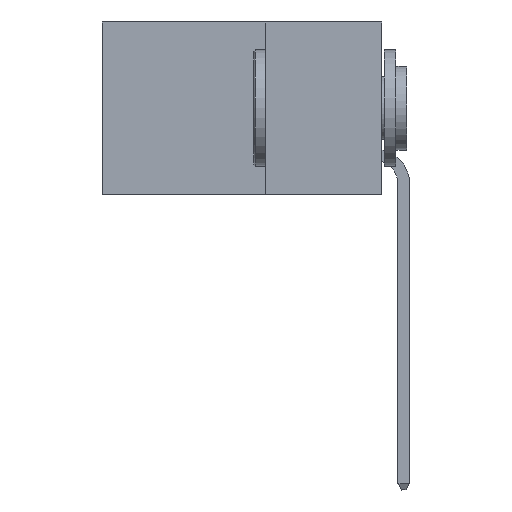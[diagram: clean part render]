
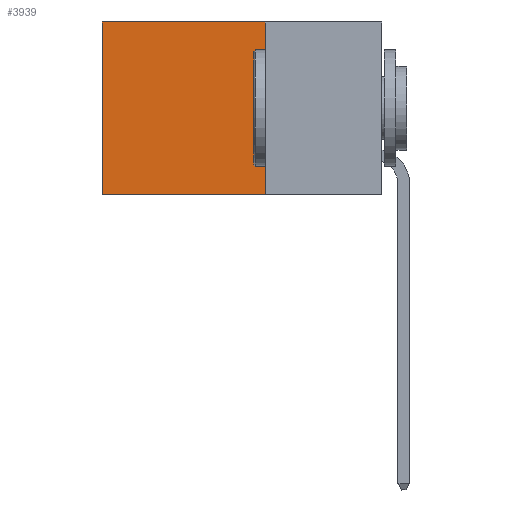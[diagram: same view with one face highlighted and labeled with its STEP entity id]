
A CAD part, left-side view. The second image highlights one B-rep face of the part: STEP entity #3939.
In plain terms, the highlighted planar face has unit normal (-1, 0, 0).
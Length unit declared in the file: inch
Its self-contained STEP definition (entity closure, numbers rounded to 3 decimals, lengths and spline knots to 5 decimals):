
#18 = CARTESIAN_POINT ( 'NONE',  ( 0.2875, 0.25, 0. ) ) ;
#191 = DIRECTION ( 'NONE',  ( 0., 0., -1. ) ) ;
#326 = DIRECTION ( 'NONE',  ( 0., 1., 0. ) ) ;
#1387 = CARTESIAN_POINT ( 'NONE',  ( 0.2875, 0.6, 0. ) ) ;
#1940 = ORIENTED_EDGE ( 'NONE', *, *, #3908, .F. ) ;
#2828 = EDGE_CURVE ( 'NONE', #11890, #6327, #3169, .T. ) ;
#2958 = EDGE_CURVE ( 'NONE', #12188, #11890, #14932, .T. ) ;
#3169 = LINE ( 'NONE', #1387, #8463 ) ;
#3596 = ORIENTED_EDGE ( 'NONE', *, *, #2958, .T. ) ;
#3908 = EDGE_CURVE ( 'NONE', #12188, #13177, #7261, .T. ) ;
#3912 = CARTESIAN_POINT ( 'NONE',  ( 0.2875, 0.6, 0. ) ) ;
#3939 = ADVANCED_FACE ( 'NONE', ( #4134 ), #12779, .F. ) ;
#4134 = FACE_OUTER_BOUND ( 'NONE', #4373, .T. ) ;
#4373 = EDGE_LOOP ( 'NONE', ( #7343, #8391, #1940, #3596 ) ) ;
#4452 = EDGE_CURVE ( 'NONE', #13177, #6327, #12382, .T. ) ;
#5087 = DIRECTION ( 'NONE',  ( 0., 0., -1. ) ) ;
#6280 = VECTOR ( 'NONE', #191, 39.37008 ) ;
#6327 = VERTEX_POINT ( 'NONE', #12019 ) ;
#6412 = CARTESIAN_POINT ( 'NONE',  ( 0.2875, 0.25, 0. ) ) ;
#6485 = VECTOR ( 'NONE', #326, 39.37008 ) ;
#7078 = CARTESIAN_POINT ( 'NONE',  ( 0.2875, 0.25, 0. ) ) ;
#7261 = LINE ( 'NONE', #6412, #6280 ) ;
#7343 = ORIENTED_EDGE ( 'NONE', *, *, #2828, .T. ) ;
#8306 = DIRECTION ( 'NONE',  ( 0., 1., 0. ) ) ;
#8391 = ORIENTED_EDGE ( 'NONE', *, *, #4452, .F. ) ;
#8463 = VECTOR ( 'NONE', #5087, 39.37008 ) ;
#9861 = CARTESIAN_POINT ( 'NONE',  ( 0.2875, 0.25, -0.37 ) ) ;
#10328 = CARTESIAN_POINT ( 'NONE',  ( 0.2875, 0.25, -0.37 ) ) ;
#11086 = AXIS2_PLACEMENT_3D ( 'NONE', #18, #12561, #12605 ) ;
#11890 = VERTEX_POINT ( 'NONE', #3912 ) ;
#12019 = CARTESIAN_POINT ( 'NONE',  ( 0.2875, 0.6, -0.37 ) ) ;
#12188 = VERTEX_POINT ( 'NONE', #14685 ) ;
#12382 = LINE ( 'NONE', #10328, #6485 ) ;
#12561 = DIRECTION ( 'NONE',  ( 1., 0., 0. ) ) ;
#12605 = DIRECTION ( 'NONE',  ( 0., 0., -1. ) ) ;
#12779 = PLANE ( 'NONE',  #11086 ) ;
#13177 = VERTEX_POINT ( 'NONE', #9861 ) ;
#13382 = VECTOR ( 'NONE', #8306, 39.37008 ) ;
#14685 = CARTESIAN_POINT ( 'NONE',  ( 0.2875, 0.25, 0. ) ) ;
#14932 = LINE ( 'NONE', #7078, #13382 ) ;
